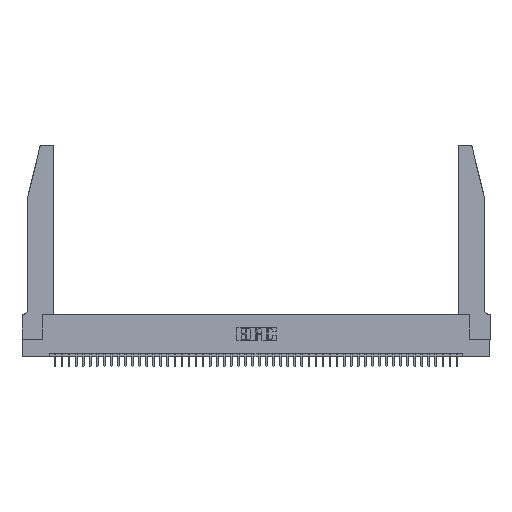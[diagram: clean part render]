
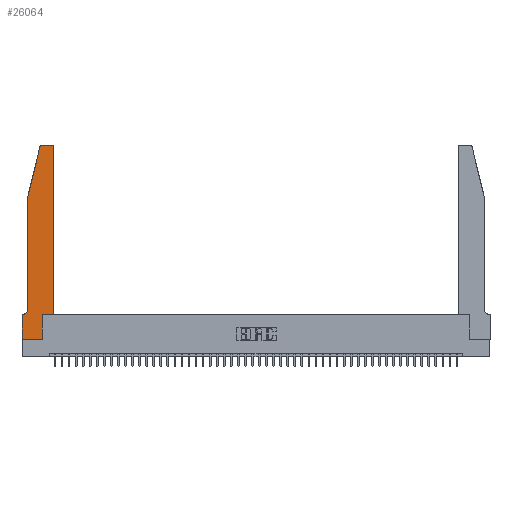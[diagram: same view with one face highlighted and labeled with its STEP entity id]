
A CAD part, top view. The second image highlights one B-rep face of the part: STEP entity #26064.
In plain terms, the highlighted planar face has unit normal (0, 0, 1).
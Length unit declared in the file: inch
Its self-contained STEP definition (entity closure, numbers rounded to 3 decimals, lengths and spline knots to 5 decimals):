
#31 = EDGE_CURVE ( 'NONE', #8094, #45967, #44454, .T. ) ;
#274 = VERTEX_POINT ( 'NONE', #40253 ) ;
#667 = VECTOR ( 'NONE', #9546, 39.37008 ) ;
#1133 = CARTESIAN_POINT ( 'NONE',  ( 0.0755, 0.35, 0.37 ) ) ;
#1582 = EDGE_CURVE ( 'NONE', #38295, #274, #20035, .T. ) ;
#1764 = CARTESIAN_POINT ( 'NONE',  ( 0.0755, 0.42, 0.37 ) ) ;
#1864 = LINE ( 'NONE', #5765, #667 ) ;
#1872 = DIRECTION ( 'NONE',  ( -1., 0., 0. ) ) ;
#4078 = EDGE_CURVE ( 'NONE', #45967, #7920, #14676, .T. ) ;
#4397 = CARTESIAN_POINT ( 'NONE',  ( 0.284, 2.75, 0.37 ) ) ;
#4954 = DIRECTION ( 'NONE',  ( -1., 0., 0. ) ) ;
#5737 = EDGE_CURVE ( 'NONE', #274, #8094, #15744, .T. ) ;
#5765 = CARTESIAN_POINT ( 'NONE',  ( 0.0755, 2., 0.37 ) ) ;
#6849 = CARTESIAN_POINT ( 'NONE',  ( 0.4505, 0.35, 0.37 ) ) ;
#7118 = CARTESIAN_POINT ( 'NONE',  ( 0.4505, 2.72, 0.37 ) ) ;
#7920 = VERTEX_POINT ( 'NONE', #11156 ) ;
#8094 = VERTEX_POINT ( 'NONE', #4397 ) ;
#8882 = DIRECTION ( 'NONE',  ( 0., 0., 1. ) ) ;
#9126 = VERTEX_POINT ( 'NONE', #10040 ) ;
#9546 = DIRECTION ( 'NONE',  ( 0., -1., 0. ) ) ;
#9711 = VECTOR ( 'NONE', #11324, 39.37008 ) ;
#9910 = AXIS2_PLACEMENT_3D ( 'NONE', #36637, #14576, #40357 ) ;
#10040 = CARTESIAN_POINT ( 'NONE',  ( 0.2865, 0.35, 0.37 ) ) ;
#11156 = CARTESIAN_POINT ( 'NONE',  ( 0.0755, 2., 0.37 ) ) ;
#11324 = DIRECTION ( 'NONE',  ( 0., 1., 0. ) ) ;
#11449 = CARTESIAN_POINT ( 'NONE',  ( 0.2865, 0., 0.37 ) ) ;
#11599 = ORIENTED_EDGE ( 'NONE', *, *, #4078, .T. ) ;
#12144 = VERTEX_POINT ( 'NONE', #1764 ) ;
#12720 = VERTEX_POINT ( 'NONE', #31168 ) ;
#13004 = VERTEX_POINT ( 'NONE', #6849 ) ;
#14050 = DIRECTION ( 'NONE',  ( 1., 0., 0. ) ) ;
#14576 = DIRECTION ( 'NONE',  ( 0., 0., 1. ) ) ;
#14676 = LINE ( 'NONE', #17536, #23336 ) ;
#15744 = LINE ( 'NONE', #27228, #24365 ) ;
#16419 = DIRECTION ( 'NONE',  ( 0., 0., 1. ) ) ;
#16853 = EDGE_CURVE ( 'NONE', #39915, #21905, #21374, .T. ) ;
#17492 = EDGE_CURVE ( 'NONE', #12720, #39915, #43321, .T. ) ;
#17536 = CARTESIAN_POINT ( 'NONE',  ( 0.0755, 2., 0.37 ) ) ;
#18564 = CIRCLE ( 'NONE', #26167, 0.07 ) ;
#18768 = ORIENTED_EDGE ( 'NONE', *, *, #43193, .T. ) ;
#19778 = VECTOR ( 'NONE', #14050, 39.37008 ) ;
#20035 = CIRCLE ( 'NONE', #43807, 0.03 ) ;
#20093 = AXIS2_PLACEMENT_3D ( 'NONE', #38490, #16419, #42214 ) ;
#20653 = EDGE_CURVE ( 'NONE', #9126, #13004, #29580, .T. ) ;
#21238 = DIRECTION ( 'NONE',  ( -0.239, -0.971, 0. ) ) ;
#21374 = LINE ( 'NONE', #33887, #30033 ) ;
#21543 = ORIENTED_EDGE ( 'NONE', *, *, #47044, .T. ) ;
#21905 = VERTEX_POINT ( 'NONE', #46573 ) ;
#22226 = DIRECTION ( 'NONE',  ( 0., 1., 0. ) ) ;
#22580 = ORIENTED_EDGE ( 'NONE', *, *, #17492, .T. ) ;
#22939 = DIRECTION ( 'NONE',  ( 0., -1., 0. ) ) ;
#23336 = VECTOR ( 'NONE', #21238, 39.37008 ) ;
#24228 = DIRECTION ( 'NONE',  ( 0., 0., -1. ) ) ;
#24365 = VECTOR ( 'NONE', #45666, 39.37008 ) ;
#25662 = VECTOR ( 'NONE', #22226, 39.37008 ) ;
#25756 = ORIENTED_EDGE ( 'NONE', *, *, #1582, .T. ) ;
#25840 = CARTESIAN_POINT ( 'NONE',  ( 0.25487, 2.72718, 0.37 ) ) ;
#26015 = ORIENTED_EDGE ( 'NONE', *, *, #20653, .T. ) ;
#26064 = ADVANCED_FACE ( 'NONE', ( #33634 ), #29238, .T. ) ;
#26167 = AXIS2_PLACEMENT_3D ( 'NONE', #46387, #24228, #1872 ) ;
#27094 = VECTOR ( 'NONE', #43698, 39.37008 ) ;
#27228 = CARTESIAN_POINT ( 'NONE',  ( 0.2605, 2.75, 0.37 ) ) ;
#28254 = LINE ( 'NONE', #37152, #9711 ) ;
#28691 = CARTESIAN_POINT ( 'NONE',  ( 0., 0., 0.37 ) ) ;
#29238 = PLANE ( 'NONE',  #9910 ) ;
#29580 = LINE ( 'NONE', #47155, #19778 ) ;
#30033 = VECTOR ( 'NONE', #22939, 39.37008 ) ;
#30416 = ORIENTED_EDGE ( 'NONE', *, *, #16853, .T. ) ;
#30616 = EDGE_CURVE ( 'NONE', #12144, #12720, #18564, .T. ) ;
#30933 = VERTEX_POINT ( 'NONE', #11449 ) ;
#31049 = CARTESIAN_POINT ( 'NONE',  ( 0.4205, 2.72, 0.37 ) ) ;
#31168 = CARTESIAN_POINT ( 'NONE',  ( 0.0055, 0.35, 0.37 ) ) ;
#33634 = FACE_OUTER_BOUND ( 'NONE', #45838, .T. ) ;
#33887 = CARTESIAN_POINT ( 'NONE',  ( 0., 0., 0.37 ) ) ;
#34326 = LINE ( 'NONE', #44331, #25662 ) ;
#34766 = DIRECTION ( 'NONE',  ( 1., 0., 0. ) ) ;
#35591 = ORIENTED_EDGE ( 'NONE', *, *, #31, .T. ) ;
#36637 = CARTESIAN_POINT ( 'NONE',  ( 0., 0.35, 0.37 ) ) ;
#36904 = LINE ( 'NONE', #28691, #27094 ) ;
#37152 = CARTESIAN_POINT ( 'NONE',  ( 0.4505, 0.35, 0.37 ) ) ;
#38295 = VERTEX_POINT ( 'NONE', #7118 ) ;
#38490 = CARTESIAN_POINT ( 'NONE',  ( 0.284, 2.72, 0.37 ) ) ;
#38717 = EDGE_CURVE ( 'NONE', #7920, #12144, #1864, .T. ) ;
#39147 = ORIENTED_EDGE ( 'NONE', *, *, #30616, .T. ) ;
#39915 = VERTEX_POINT ( 'NONE', #47137 ) ;
#40253 = CARTESIAN_POINT ( 'NONE',  ( 0.4205, 2.75, 0.37 ) ) ;
#40357 = DIRECTION ( 'NONE',  ( 1., 0., 0. ) ) ;
#40428 = ORIENTED_EDGE ( 'NONE', *, *, #38717, .T. ) ;
#41324 = ORIENTED_EDGE ( 'NONE', *, *, #5737, .T. ) ;
#42153 = VECTOR ( 'NONE', #4954, 39.37008 ) ;
#42214 = DIRECTION ( 'NONE',  ( 1., 0., 0. ) ) ;
#43193 = EDGE_CURVE ( 'NONE', #13004, #38295, #28254, .T. ) ;
#43321 = LINE ( 'NONE', #1133, #42153 ) ;
#43698 = DIRECTION ( 'NONE',  ( 1., 0., 0. ) ) ;
#43807 = AXIS2_PLACEMENT_3D ( 'NONE', #31049, #8882, #34766 ) ;
#44260 = EDGE_CURVE ( 'NONE', #21905, #30933, #36904, .T. ) ;
#44331 = CARTESIAN_POINT ( 'NONE',  ( 0.2865, 0.35, 0.37 ) ) ;
#44454 = CIRCLE ( 'NONE', #20093, 0.03 ) ;
#44853 = ORIENTED_EDGE ( 'NONE', *, *, #44260, .T. ) ;
#45666 = DIRECTION ( 'NONE',  ( -1., 0., 0. ) ) ;
#45838 = EDGE_LOOP ( 'NONE', ( #41324, #35591, #11599, #40428, #39147, #22580, #30416, #44853, #21543, #26015, #18768, #25756 ) ) ;
#45967 = VERTEX_POINT ( 'NONE', #25840 ) ;
#46387 = CARTESIAN_POINT ( 'NONE',  ( 0.0055, 0.42, 0.37 ) ) ;
#46573 = CARTESIAN_POINT ( 'NONE',  ( 0., 0., 0.37 ) ) ;
#47044 = EDGE_CURVE ( 'NONE', #30933, #9126, #34326, .T. ) ;
#47137 = CARTESIAN_POINT ( 'NONE',  ( 0., 0.35, 0.37 ) ) ;
#47155 = CARTESIAN_POINT ( 'NONE',  ( 0.4505, 0.35, 0.37 ) ) ;
